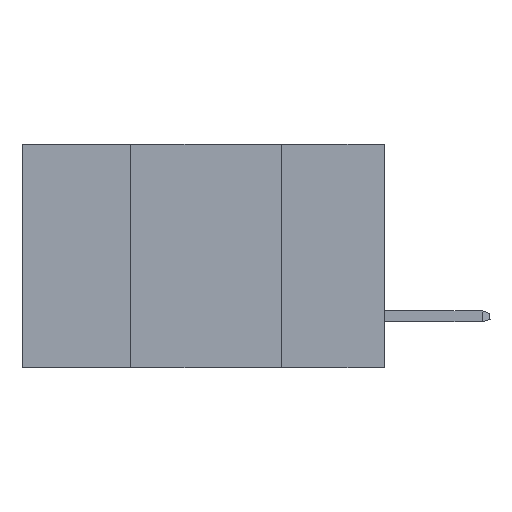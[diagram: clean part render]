
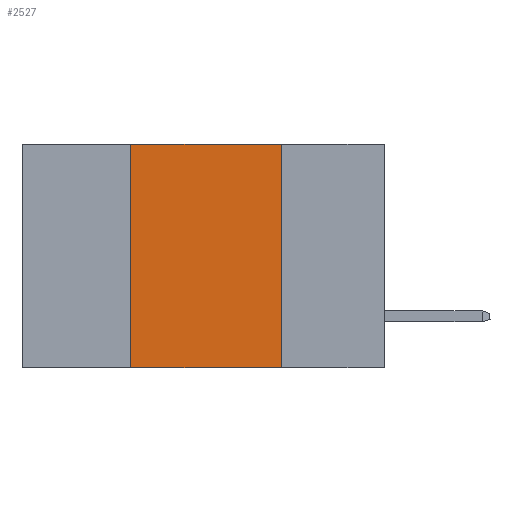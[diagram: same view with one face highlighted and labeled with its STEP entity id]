
A CAD part, left-side view. The second image highlights one B-rep face of the part: STEP entity #2527.
In plain terms, the highlighted planar face has unit normal (-1, 0, 0).
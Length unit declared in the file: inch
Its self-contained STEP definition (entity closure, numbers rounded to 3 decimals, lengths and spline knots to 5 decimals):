
#87 = FACE_OUTER_BOUND ( 'NONE', #27870, .T. ) ;
#158 = VERTEX_POINT ( 'NONE', #22084 ) ;
#1705 = PLANE ( 'NONE',  #24792 ) ;
#1952 = CARTESIAN_POINT ( 'NONE',  ( 0., 0.42, 0. ) ) ;
#2202 = VECTOR ( 'NONE', #13905, 39.37008 ) ;
#2527 = ADVANCED_FACE ( 'NONE', ( #87 ), #1705, .F. ) ;
#3032 = ORIENTED_EDGE ( 'NONE', *, *, #31308, .F. ) ;
#4589 = EDGE_CURVE ( 'NONE', #11389, #13299, #27999, .T. ) ;
#5432 = LINE ( 'NONE', #12313, #22083 ) ;
#6967 = CARTESIAN_POINT ( 'NONE',  ( 0., 0.6, -0.37 ) ) ;
#7385 = ORIENTED_EDGE ( 'NONE', *, *, #10831, .F. ) ;
#7938 = CARTESIAN_POINT ( 'NONE',  ( 0., 0.42, -0.37 ) ) ;
#9244 = DIRECTION ( 'NONE',  ( 1., 0., 0. ) ) ;
#9391 = DIRECTION ( 'NONE',  ( 0., -1., 0. ) ) ;
#10672 = VECTOR ( 'NONE', #9391, 39.37008 ) ;
#10831 = EDGE_CURVE ( 'NONE', #13299, #14050, #29278, .T. ) ;
#11389 = VERTEX_POINT ( 'NONE', #7938 ) ;
#11802 = LINE ( 'NONE', #6967, #10672 ) ;
#12111 = ORIENTED_EDGE ( 'NONE', *, *, #4589, .F. ) ;
#12313 = CARTESIAN_POINT ( 'NONE',  ( 0., 0.17, 0. ) ) ;
#13299 = VERTEX_POINT ( 'NONE', #18547 ) ;
#13457 = CARTESIAN_POINT ( 'NONE',  ( 0., 0.6, 0. ) ) ;
#13905 = DIRECTION ( 'NONE',  ( 0., 0., 1. ) ) ;
#14050 = VERTEX_POINT ( 'NONE', #23626 ) ;
#16362 = VECTOR ( 'NONE', #28013, 39.37008 ) ;
#16977 = DIRECTION ( 'NONE',  ( 0., 0., -1. ) ) ;
#17278 = EDGE_CURVE ( 'NONE', #11389, #158, #11802, .T. ) ;
#18104 = ORIENTED_EDGE ( 'NONE', *, *, #17278, .T. ) ;
#18547 = CARTESIAN_POINT ( 'NONE',  ( 0., 0.42, 0. ) ) ;
#18645 = CARTESIAN_POINT ( 'NONE',  ( 0., 0.6, 0. ) ) ;
#22083 = VECTOR ( 'NONE', #16977, 39.37008 ) ;
#22084 = CARTESIAN_POINT ( 'NONE',  ( 0., 0.17, -0.37 ) ) ;
#23557 = DIRECTION ( 'NONE',  ( 0., 0., -1. ) ) ;
#23626 = CARTESIAN_POINT ( 'NONE',  ( 0., 0.17, 0. ) ) ;
#24792 = AXIS2_PLACEMENT_3D ( 'NONE', #18645, #9244, #23557 ) ;
#27870 = EDGE_LOOP ( 'NONE', ( #3032, #7385, #12111, #18104 ) ) ;
#27999 = LINE ( 'NONE', #1952, #2202 ) ;
#28013 = DIRECTION ( 'NONE',  ( 0., -1., 0. ) ) ;
#29278 = LINE ( 'NONE', #13457, #16362 ) ;
#31308 = EDGE_CURVE ( 'NONE', #14050, #158, #5432, .T. ) ;
